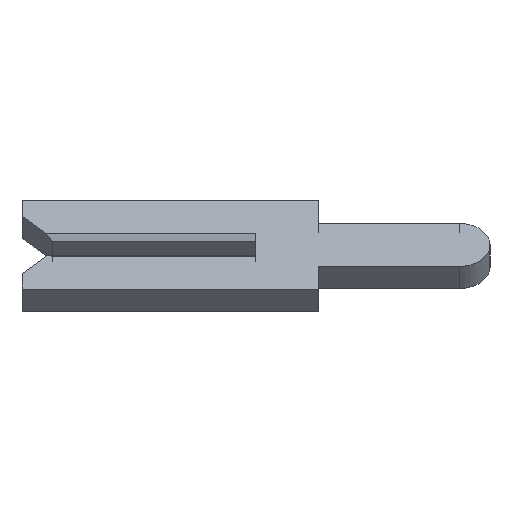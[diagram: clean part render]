
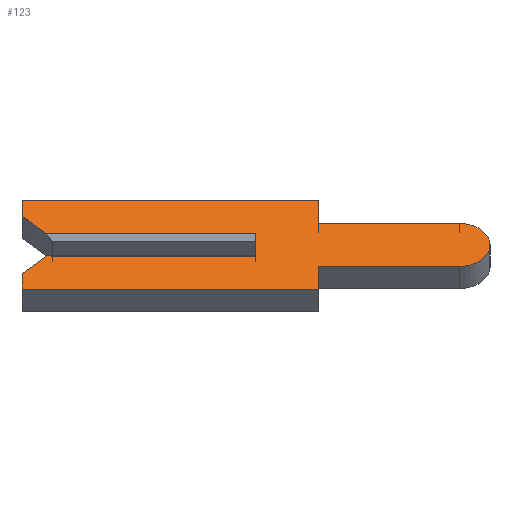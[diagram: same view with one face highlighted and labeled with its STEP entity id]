
A CAD part, left-side view. The second image highlights one B-rep face of the part: STEP entity #123.
In plain terms, the highlighted face is planar.
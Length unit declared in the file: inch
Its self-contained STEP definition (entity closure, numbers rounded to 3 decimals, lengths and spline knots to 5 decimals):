
#29 = CARTESIAN_POINT ( 'NONE',  ( -0.01, 0.15, -0.026 ) ) ;
#66 = VERTEX_POINT ( 'NONE', #629 ) ;
#68 = VERTEX_POINT ( 'NONE', #1615 ) ;
#84 = VECTOR ( 'NONE', #1177, 39.37008 ) ;
#101 = DIRECTION ( 'NONE',  ( 1., 0., 0. ) ) ;
#102 = EDGE_CURVE ( 'NONE', #1323, #68, #1686, .T. ) ;
#122 = LINE ( 'NONE', #483, #84 ) ;
#123 = ADVANCED_FACE ( 'NONE', ( #641 ), #359, .F. ) ;
#124 = VECTOR ( 'NONE', #1574, 39.37008 ) ;
#128 = ORIENTED_EDGE ( 'NONE', *, *, #1219, .F. ) ;
#146 = CARTESIAN_POINT ( 'NONE',  ( -0.01, -0.1305, -0.01 ) ) ;
#165 = VECTOR ( 'NONE', #995, 39.37008 ) ;
#166 = CARTESIAN_POINT ( 'NONE',  ( -0.01, -0.04, 0.0195 ) ) ;
#169 = VERTEX_POINT ( 'NONE', #1358 ) ;
#176 = EDGE_CURVE ( 'NONE', #1277, #660, #258, .T. ) ;
#223 = ORIENTED_EDGE ( 'NONE', *, *, #1053, .F. ) ;
#241 = DIRECTION ( 'NONE',  ( 0., 0., 1. ) ) ;
#247 = ORIENTED_EDGE ( 'NONE', *, *, #392, .F. ) ;
#249 = DIRECTION ( 'NONE',  ( 0., 0., -1. ) ) ;
#258 = LINE ( 'NONE', #1222, #830 ) ;
#302 = LINE ( 'NONE', #166, #915 ) ;
#359 = PLANE ( 'NONE',  #1348 ) ;
#372 = EDGE_CURVE ( 'NONE', #1203, #880, #1489, .T. ) ;
#374 = LINE ( 'NONE', #1530, #657 ) ;
#377 = ORIENTED_EDGE ( 'NONE', *, *, #759, .T. ) ;
#390 = DIRECTION ( 'NONE',  ( 1., 0., 0. ) ) ;
#392 = EDGE_CURVE ( 'NONE', #1621, #949, #374, .T. ) ;
#397 = VECTOR ( 'NONE', #783, 39.37008 ) ;
#401 = ORIENTED_EDGE ( 'NONE', *, *, #990, .F. ) ;
#441 = DIRECTION ( 'NONE',  ( 0., 0., 1. ) ) ;
#476 = AXIS2_PLACEMENT_3D ( 'NONE', #1085, #390, #249 ) ;
#483 = CARTESIAN_POINT ( 'NONE',  ( -0.01, 0.15, 0.04 ) ) ;
#490 = CARTESIAN_POINT ( 'NONE',  ( -0.01, -0.04, 0.04 ) ) ;
#502 = LINE ( 'NONE', #146, #124 ) ;
#505 = CARTESIAN_POINT ( 'NONE',  ( -0.01, -0.04, -0.04 ) ) ;
#567 = LINE ( 'NONE', #1320, #397 ) ;
#577 = EDGE_CURVE ( 'NONE', #169, #1346, #725, .T. ) ;
#586 = DIRECTION ( 'NONE',  ( 0., 1., 0. ) ) ;
#600 = CARTESIAN_POINT ( 'NONE',  ( -0.01, -0.04, -0.0195 ) ) ;
#621 = VERTEX_POINT ( 'NONE', #1567 ) ;
#629 = CARTESIAN_POINT ( 'NONE',  ( -0.01, 0.134, -0.01 ) ) ;
#637 = CARTESIAN_POINT ( 'NONE',  ( -0.01, -0.04, -0.04 ) ) ;
#641 = FACE_OUTER_BOUND ( 'NONE', #1665, .T. ) ;
#657 = VECTOR ( 'NONE', #1508, 39.37008 ) ;
#660 = VERTEX_POINT ( 'NONE', #29 ) ;
#664 = ORIENTED_EDGE ( 'NONE', *, *, #1119, .F. ) ;
#725 = LINE ( 'NONE', #1280, #755 ) ;
#730 = ORIENTED_EDGE ( 'NONE', *, *, #764, .F. ) ;
#742 = CARTESIAN_POINT ( 'NONE',  ( -0.01, 0.15, 0.04 ) ) ;
#755 = VECTOR ( 'NONE', #441, 39.37008 ) ;
#759 = EDGE_CURVE ( 'NONE', #621, #1346, #1058, .T. ) ;
#764 = EDGE_CURVE ( 'NONE', #66, #169, #502, .T. ) ;
#767 = CARTESIAN_POINT ( 'NONE',  ( -0.01, -0.04, 0.04 ) ) ;
#783 = DIRECTION ( 'NONE',  ( 0., 0.707, 0.707 ) ) ;
#830 = VECTOR ( 'NONE', #241, 39.37008 ) ;
#845 = CARTESIAN_POINT ( 'NONE',  ( -0.01, 0.15, 0.01 ) ) ;
#856 = EDGE_CURVE ( 'NONE', #880, #904, #1370, .T. ) ;
#880 = VERTEX_POINT ( 'NONE', #1306 ) ;
#899 = VECTOR ( 'NONE', #1369, 39.37008 ) ;
#904 = VERTEX_POINT ( 'NONE', #1444 ) ;
#915 = VECTOR ( 'NONE', #1597, 39.37008 ) ;
#919 = DIRECTION ( 'NONE',  ( 0., 0., -1. ) ) ;
#949 = VERTEX_POINT ( 'NONE', #742 ) ;
#986 = VECTOR ( 'NONE', #586, 39.37008 ) ;
#990 = EDGE_CURVE ( 'NONE', #68, #1203, #302, .T. ) ;
#995 = DIRECTION ( 'NONE',  ( 0., -1., 0. ) ) ;
#1053 = EDGE_CURVE ( 'NONE', #949, #1323, #122, .T. ) ;
#1058 = LINE ( 'NONE', #845, #165 ) ;
#1085 = CARTESIAN_POINT ( 'NONE',  ( -0.01, -0.1305, 0. ) ) ;
#1094 = LINE ( 'NONE', #637, #1685 ) ;
#1116 = ORIENTED_EDGE ( 'NONE', *, *, #102, .F. ) ;
#1119 = EDGE_CURVE ( 'NONE', #904, #1375, #1094, .T. ) ;
#1177 = DIRECTION ( 'NONE',  ( 0., -1., 0. ) ) ;
#1190 = CARTESIAN_POINT ( 'NONE',  ( -0.01, -0.1305, 0.0195 ) ) ;
#1196 = EDGE_CURVE ( 'NONE', #621, #1621, #567, .T. ) ;
#1203 = VERTEX_POINT ( 'NONE', #1190 ) ;
#1219 = EDGE_CURVE ( 'NONE', #660, #66, #1545, .T. ) ;
#1222 = CARTESIAN_POINT ( 'NONE',  ( -0.01, 0.15, -0.026 ) ) ;
#1244 = ORIENTED_EDGE ( 'NONE', *, *, #1353, .F. ) ;
#1277 = VERTEX_POINT ( 'NONE', #1345 ) ;
#1280 = CARTESIAN_POINT ( 'NONE',  ( -0.01, 0., 0.0065 ) ) ;
#1292 = LINE ( 'NONE', #1803, #899 ) ;
#1306 = CARTESIAN_POINT ( 'NONE',  ( -0.01, -0.1305, -0.0195 ) ) ;
#1320 = CARTESIAN_POINT ( 'NONE',  ( -0.01, 0.1305, 0.0065 ) ) ;
#1323 = VERTEX_POINT ( 'NONE', #490 ) ;
#1330 = CARTESIAN_POINT ( 'NONE',  ( -0.01, 0.1305, -0.0065 ) ) ;
#1339 = DIRECTION ( 'NONE',  ( 0., -0.707, 0.707 ) ) ;
#1342 = CARTESIAN_POINT ( 'NONE',  ( -0.01, -0.1305, 0. ) ) ;
#1345 = CARTESIAN_POINT ( 'NONE',  ( -0.01, 0.15, -0.04 ) ) ;
#1346 = VERTEX_POINT ( 'NONE', #1670 ) ;
#1348 = AXIS2_PLACEMENT_3D ( 'NONE', #1342, #101, #1796 ) ;
#1353 = EDGE_CURVE ( 'NONE', #1375, #1277, #1292, .T. ) ;
#1358 = CARTESIAN_POINT ( 'NONE',  ( -0.01, 0., -0.01 ) ) ;
#1369 = DIRECTION ( 'NONE',  ( 0., 1., 0. ) ) ;
#1370 = LINE ( 'NONE', #600, #986 ) ;
#1375 = VERTEX_POINT ( 'NONE', #505 ) ;
#1444 = CARTESIAN_POINT ( 'NONE',  ( -0.01, -0.04, -0.0195 ) ) ;
#1448 = ORIENTED_EDGE ( 'NONE', *, *, #372, .F. ) ;
#1485 = DIRECTION ( 'NONE',  ( 0., 0., -1. ) ) ;
#1488 = VECTOR ( 'NONE', #1339, 39.37008 ) ;
#1489 = CIRCLE ( 'NONE', #476, 0.0195 ) ;
#1508 = DIRECTION ( 'NONE',  ( 0., 0., 1. ) ) ;
#1515 = ORIENTED_EDGE ( 'NONE', *, *, #577, .F. ) ;
#1526 = CARTESIAN_POINT ( 'NONE',  ( -0.01, 0.15, 0.026 ) ) ;
#1530 = CARTESIAN_POINT ( 'NONE',  ( -0.01, 0.15, 0.026 ) ) ;
#1545 = LINE ( 'NONE', #1330, #1488 ) ;
#1554 = ORIENTED_EDGE ( 'NONE', *, *, #176, .F. ) ;
#1567 = CARTESIAN_POINT ( 'NONE',  ( -0.01, 0.134, 0.01 ) ) ;
#1574 = DIRECTION ( 'NONE',  ( 0., -1., 0. ) ) ;
#1580 = ORIENTED_EDGE ( 'NONE', *, *, #856, .F. ) ;
#1597 = DIRECTION ( 'NONE',  ( 0., -1., 0. ) ) ;
#1598 = ORIENTED_EDGE ( 'NONE', *, *, #1196, .F. ) ;
#1615 = CARTESIAN_POINT ( 'NONE',  ( -0.01, -0.04, 0.0195 ) ) ;
#1621 = VERTEX_POINT ( 'NONE', #1526 ) ;
#1640 = VECTOR ( 'NONE', #919, 39.37008 ) ;
#1665 = EDGE_LOOP ( 'NONE', ( #377, #1515, #730, #128, #1554, #1244, #664, #1580, #1448, #401, #1116, #223, #247, #1598 ) ) ;
#1670 = CARTESIAN_POINT ( 'NONE',  ( -0.01, 0., 0.01 ) ) ;
#1685 = VECTOR ( 'NONE', #1485, 39.37008 ) ;
#1686 = LINE ( 'NONE', #767, #1640 ) ;
#1796 = DIRECTION ( 'NONE',  ( 0., 0., -1. ) ) ;
#1803 = CARTESIAN_POINT ( 'NONE',  ( -0.01, 0.15, -0.04 ) ) ;
